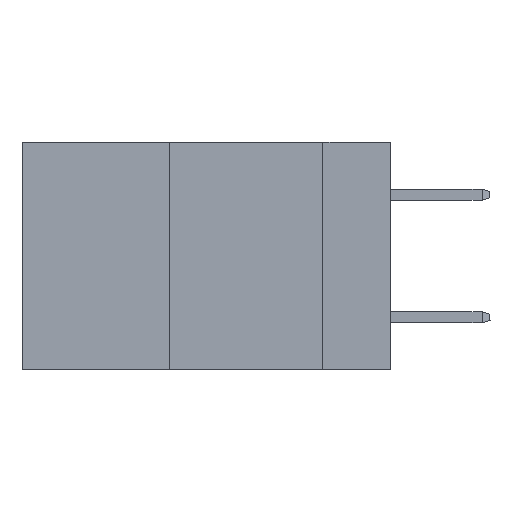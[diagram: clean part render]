
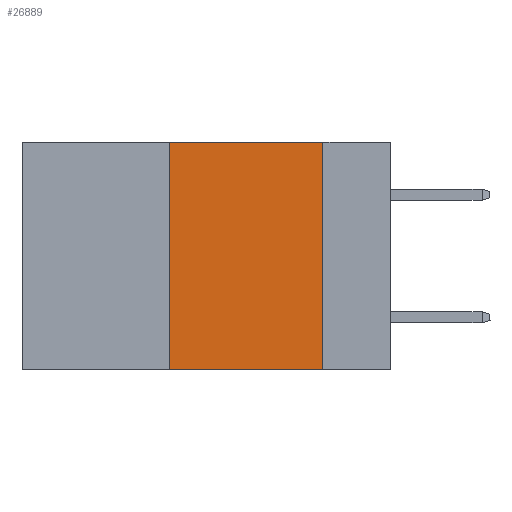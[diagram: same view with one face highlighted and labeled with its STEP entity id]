
A CAD part, left-side view. The second image highlights one B-rep face of the part: STEP entity #26889.
In plain terms, the highlighted planar face has unit normal (-1, 0, 0).
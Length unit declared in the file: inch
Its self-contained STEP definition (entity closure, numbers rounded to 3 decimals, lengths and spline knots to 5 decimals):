
#101 = EDGE_CURVE ( 'NONE', #28121, #27496, #10270, .T. ) ;
#627 = ORIENTED_EDGE ( 'NONE', *, *, #101, .F. ) ;
#766 = DIRECTION ( 'NONE',  ( 0., 0., -1. ) ) ;
#1252 = PLANE ( 'NONE',  #16966 ) ;
#2484 = ORIENTED_EDGE ( 'NONE', *, *, #2872, .F. ) ;
#2872 = EDGE_CURVE ( 'NONE', #16599, #17599, #13876, .T. ) ;
#2961 = FACE_OUTER_BOUND ( 'NONE', #16185, .T. ) ;
#3756 = DIRECTION ( 'NONE',  ( 1., 0., 0. ) ) ;
#4215 = LINE ( 'NONE', #25352, #25574 ) ;
#4926 = DIRECTION ( 'NONE',  ( 0., -1., 0. ) ) ;
#5254 = DIRECTION ( 'NONE',  ( 0., -1., 0. ) ) ;
#5445 = CARTESIAN_POINT ( 'NONE',  ( 0., 0.36, -0.37 ) ) ;
#6301 = CARTESIAN_POINT ( 'NONE',  ( 0., 0.11, 0. ) ) ;
#6985 = VECTOR ( 'NONE', #16850, 39.37008 ) ;
#8162 = CARTESIAN_POINT ( 'NONE',  ( 0., 0.36, 0. ) ) ;
#10270 = LINE ( 'NONE', #6301, #27103 ) ;
#13876 = LINE ( 'NONE', #16951, #6985 ) ;
#13970 = EDGE_CURVE ( 'NONE', #16599, #27496, #27540, .T. ) ;
#16185 = EDGE_LOOP ( 'NONE', ( #627, #20912, #2484, #17352 ) ) ;
#16599 = VERTEX_POINT ( 'NONE', #5445 ) ;
#16850 = DIRECTION ( 'NONE',  ( 0., 0., 1. ) ) ;
#16951 = CARTESIAN_POINT ( 'NONE',  ( 0., 0.36, 0. ) ) ;
#16966 = AXIS2_PLACEMENT_3D ( 'NONE', #21295, #3756, #21002 ) ;
#17352 = ORIENTED_EDGE ( 'NONE', *, *, #13970, .T. ) ;
#17599 = VERTEX_POINT ( 'NONE', #8162 ) ;
#18120 = CARTESIAN_POINT ( 'NONE',  ( 0., 0.6, -0.37 ) ) ;
#18814 = CARTESIAN_POINT ( 'NONE',  ( 0., 0.11, 0. ) ) ;
#20912 = ORIENTED_EDGE ( 'NONE', *, *, #21994, .F. ) ;
#21002 = DIRECTION ( 'NONE',  ( 0., 0., -1. ) ) ;
#21295 = CARTESIAN_POINT ( 'NONE',  ( 0., 0.6, 0. ) ) ;
#21994 = EDGE_CURVE ( 'NONE', #17599, #28121, #4215, .T. ) ;
#25211 = CARTESIAN_POINT ( 'NONE',  ( 0., 0.11, -0.37 ) ) ;
#25352 = CARTESIAN_POINT ( 'NONE',  ( 0., 0.6, 0. ) ) ;
#25465 = VECTOR ( 'NONE', #4926, 39.37008 ) ;
#25574 = VECTOR ( 'NONE', #5254, 39.37008 ) ;
#26889 = ADVANCED_FACE ( 'NONE', ( #2961 ), #1252, .F. ) ;
#27103 = VECTOR ( 'NONE', #766, 39.37008 ) ;
#27496 = VERTEX_POINT ( 'NONE', #25211 ) ;
#27540 = LINE ( 'NONE', #18120, #25465 ) ;
#28121 = VERTEX_POINT ( 'NONE', #18814 ) ;
